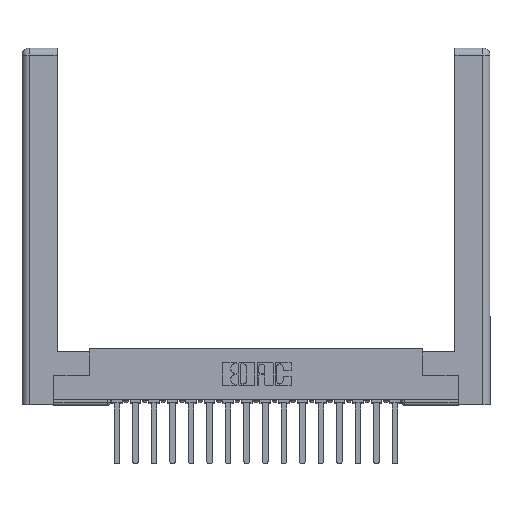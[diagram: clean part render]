
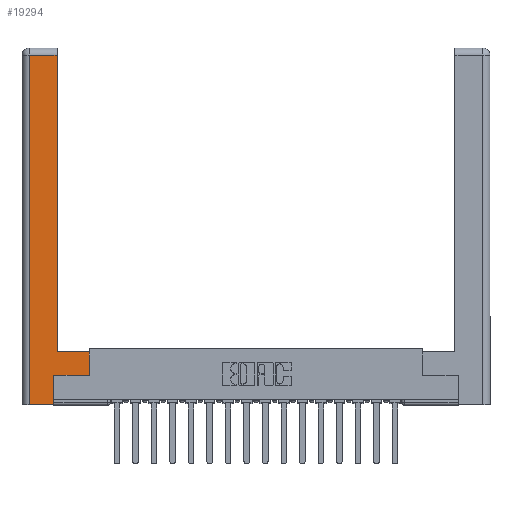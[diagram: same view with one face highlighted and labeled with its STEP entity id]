
A CAD part, top view. The second image highlights one B-rep face of the part: STEP entity #19294.
In plain terms, the highlighted planar face has unit normal (0, 0, 1).
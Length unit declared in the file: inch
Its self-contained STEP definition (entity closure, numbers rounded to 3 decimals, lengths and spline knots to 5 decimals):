
#143 = VERTEX_POINT ( 'NONE', #1776 ) ;
#244 = DIRECTION ( 'NONE',  ( 0., 1., 0. ) ) ;
#303 = VECTOR ( 'NONE', #5129, 39.37008 ) ;
#597 = LINE ( 'NONE', #3551, #14339 ) ;
#708 = LINE ( 'NONE', #8508, #2314 ) ;
#1531 = EDGE_CURVE ( 'NONE', #12938, #18947, #6391, .T. ) ;
#1776 = CARTESIAN_POINT ( 'NONE',  ( 0.0615, 2.94, 0. ) ) ;
#1851 = DIRECTION ( 'NONE',  ( 0., 1., 0. ) ) ;
#2314 = VECTOR ( 'NONE', #14661, 39.37008 ) ;
#2505 = DIRECTION ( 'NONE',  ( 0., 0., -1. ) ) ;
#2620 = EDGE_LOOP ( 'NONE', ( #6890, #13800, #5020, #6995, #13165, #6659, #19769, #17927 ) ) ;
#3162 = LINE ( 'NONE', #4921, #10498 ) ;
#3302 = VERTEX_POINT ( 'NONE', #15854 ) ;
#3551 = CARTESIAN_POINT ( 'NONE',  ( 0.0615, 0., 0. ) ) ;
#3592 = CARTESIAN_POINT ( 'NONE',  ( 0.265, 0., 0. ) ) ;
#3705 = VERTEX_POINT ( 'NONE', #5105 ) ;
#4245 = CARTESIAN_POINT ( 'NONE',  ( 0., 0., 0. ) ) ;
#4595 = DIRECTION ( 'NONE',  ( -1., 0., 0. ) ) ;
#4921 = CARTESIAN_POINT ( 'NONE',  ( 0.295, 3., 0. ) ) ;
#5020 = ORIENTED_EDGE ( 'NONE', *, *, #5688, .T. ) ;
#5105 = CARTESIAN_POINT ( 'NONE',  ( 0.265, 0.245, 0. ) ) ;
#5129 = DIRECTION ( 'NONE',  ( 0., 1., 0. ) ) ;
#5522 = CARTESIAN_POINT ( 'NONE',  ( 0.565, 0.245, 0. ) ) ;
#5688 = EDGE_CURVE ( 'NONE', #143, #3302, #597, .T. ) ;
#5799 = PLANE ( 'NONE',  #12824 ) ;
#6125 = LINE ( 'NONE', #6535, #7550 ) ;
#6391 = LINE ( 'NONE', #17367, #17212 ) ;
#6535 = CARTESIAN_POINT ( 'NONE',  ( 0.565, 0.245, 0. ) ) ;
#6659 = ORIENTED_EDGE ( 'NONE', *, *, #19000, .T. ) ;
#6890 = ORIENTED_EDGE ( 'NONE', *, *, #18544, .T. ) ;
#6960 = EDGE_CURVE ( 'NONE', #18792, #143, #12396, .T. ) ;
#6987 = EDGE_CURVE ( 'NONE', #18947, #7422, #708, .T. ) ;
#6995 = ORIENTED_EDGE ( 'NONE', *, *, #14188, .T. ) ;
#7422 = VERTEX_POINT ( 'NONE', #14737 ) ;
#7550 = VECTOR ( 'NONE', #7995, 39.37008 ) ;
#7995 = DIRECTION ( 'NONE',  ( 1., 0., 0. ) ) ;
#8508 = CARTESIAN_POINT ( 'NONE',  ( 0.295, 0.45, 0. ) ) ;
#10498 = VECTOR ( 'NONE', #1851, 39.37008 ) ;
#11085 = CARTESIAN_POINT ( 'NONE',  ( 0.0615, 2.94, 0. ) ) ;
#12396 = LINE ( 'NONE', #11085, #14449 ) ;
#12822 = DIRECTION ( 'NONE',  ( 0., -1., 0. ) ) ;
#12824 = AXIS2_PLACEMENT_3D ( 'NONE', #4245, #2505, #15037 ) ;
#12938 = VERTEX_POINT ( 'NONE', #5522 ) ;
#13165 = ORIENTED_EDGE ( 'NONE', *, *, #15836, .T. ) ;
#13223 = VECTOR ( 'NONE', #19447, 39.37008 ) ;
#13242 = CARTESIAN_POINT ( 'NONE',  ( 0.265, 0.245, 0. ) ) ;
#13506 = FACE_OUTER_BOUND ( 'NONE', #2620, .T. ) ;
#13800 = ORIENTED_EDGE ( 'NONE', *, *, #6960, .T. ) ;
#14030 = CARTESIAN_POINT ( 'NONE',  ( 0.565, 0.45, 0. ) ) ;
#14188 = EDGE_CURVE ( 'NONE', #3302, #18402, #18069, .T. ) ;
#14339 = VECTOR ( 'NONE', #12822, 39.37008 ) ;
#14449 = VECTOR ( 'NONE', #4595, 39.37008 ) ;
#14583 = LINE ( 'NONE', #13242, #303 ) ;
#14661 = DIRECTION ( 'NONE',  ( -1., 0., 0. ) ) ;
#14737 = CARTESIAN_POINT ( 'NONE',  ( 0.295, 0.45, 0. ) ) ;
#14913 = CARTESIAN_POINT ( 'NONE',  ( 0.265, 0., 0. ) ) ;
#14968 = CARTESIAN_POINT ( 'NONE',  ( 0.295, 2.94, 0. ) ) ;
#15037 = DIRECTION ( 'NONE',  ( -1., 0., 0. ) ) ;
#15836 = EDGE_CURVE ( 'NONE', #18402, #3705, #14583, .T. ) ;
#15854 = CARTESIAN_POINT ( 'NONE',  ( 0.0615, 0., 0. ) ) ;
#17212 = VECTOR ( 'NONE', #244, 39.37008 ) ;
#17367 = CARTESIAN_POINT ( 'NONE',  ( 0.565, 0.45, 0. ) ) ;
#17927 = ORIENTED_EDGE ( 'NONE', *, *, #6987, .T. ) ;
#18069 = LINE ( 'NONE', #3592, #13223 ) ;
#18402 = VERTEX_POINT ( 'NONE', #14913 ) ;
#18544 = EDGE_CURVE ( 'NONE', #7422, #18792, #3162, .T. ) ;
#18792 = VERTEX_POINT ( 'NONE', #14968 ) ;
#18947 = VERTEX_POINT ( 'NONE', #14030 ) ;
#19000 = EDGE_CURVE ( 'NONE', #3705, #12938, #6125, .T. ) ;
#19294 = ADVANCED_FACE ( 'NONE', ( #13506 ), #5799, .F. ) ;
#19447 = DIRECTION ( 'NONE',  ( 1., 0., 0. ) ) ;
#19769 = ORIENTED_EDGE ( 'NONE', *, *, #1531, .T. ) ;
